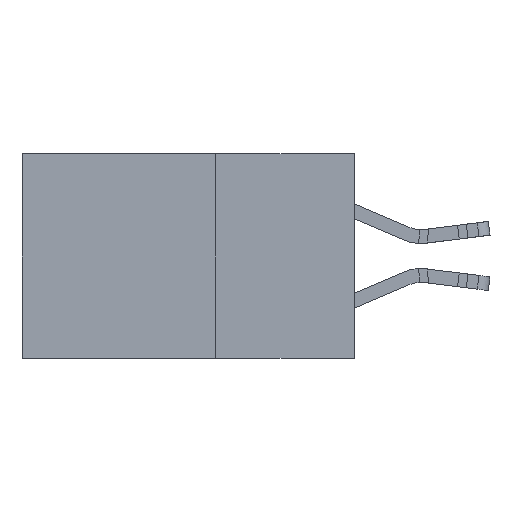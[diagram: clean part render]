
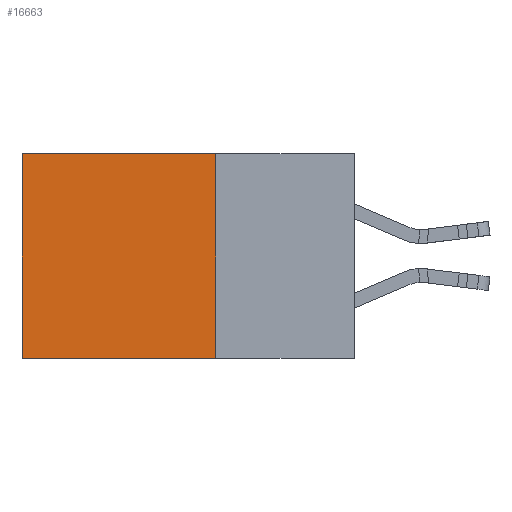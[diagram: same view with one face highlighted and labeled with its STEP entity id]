
A CAD part, left-side view. The second image highlights one B-rep face of the part: STEP entity #16663.
In plain terms, the highlighted planar face has unit normal (-1, 0, 0).
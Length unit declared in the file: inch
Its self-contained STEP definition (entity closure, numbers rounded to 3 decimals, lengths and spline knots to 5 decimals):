
#242 = VERTEX_POINT ( 'NONE', #12766 ) ;
#516 = DIRECTION ( 'NONE',  ( 0., 0., -1. ) ) ;
#1261 = LINE ( 'NONE', #14222, #22498 ) ;
#1479 = DIRECTION ( 'NONE',  ( 0., 0., -1. ) ) ;
#1963 = VECTOR ( 'NONE', #5685, 39.37008 ) ;
#3365 = FACE_OUTER_BOUND ( 'NONE', #12067, .T. ) ;
#3487 = CARTESIAN_POINT ( 'NONE',  ( 0.2615, 0.25, -0.37 ) ) ;
#3983 = EDGE_CURVE ( 'NONE', #13902, #20471, #5508, .T. ) ;
#5508 = LINE ( 'NONE', #19855, #7546 ) ;
#5685 = DIRECTION ( 'NONE',  ( 0., 1., 0. ) ) ;
#6141 = AXIS2_PLACEMENT_3D ( 'NONE', #3487, #16560, #1479 ) ;
#6153 = CARTESIAN_POINT ( 'NONE',  ( 0.2615, 0.6, -0.37 ) ) ;
#7269 = PLANE ( 'NONE',  #6141 ) ;
#7455 = LINE ( 'NONE', #9456, #1963 ) ;
#7546 = VECTOR ( 'NONE', #18314, 39.37008 ) ;
#8210 = LINE ( 'NONE', #17981, #14396 ) ;
#9023 = EDGE_CURVE ( 'NONE', #242, #16367, #7455, .T. ) ;
#9061 = EDGE_CURVE ( 'NONE', #13902, #242, #8210, .T. ) ;
#9456 = CARTESIAN_POINT ( 'NONE',  ( 0.2615, 0.25, -0.37 ) ) ;
#12067 = EDGE_LOOP ( 'NONE', ( #21824, #14579, #18912, #21619 ) ) ;
#12232 = CARTESIAN_POINT ( 'NONE',  ( 0.2615, 0.25, 0. ) ) ;
#12766 = CARTESIAN_POINT ( 'NONE',  ( 0.2615, 0.25, -0.37 ) ) ;
#13902 = VERTEX_POINT ( 'NONE', #12232 ) ;
#14077 = EDGE_CURVE ( 'NONE', #20471, #16367, #1261, .T. ) ;
#14222 = CARTESIAN_POINT ( 'NONE',  ( 0.2615, 0.6, -0.37 ) ) ;
#14396 = VECTOR ( 'NONE', #516, 39.37008 ) ;
#14579 = ORIENTED_EDGE ( 'NONE', *, *, #9023, .F. ) ;
#16367 = VERTEX_POINT ( 'NONE', #6153 ) ;
#16560 = DIRECTION ( 'NONE',  ( 1., 0., 0. ) ) ;
#16663 = ADVANCED_FACE ( 'NONE', ( #3365 ), #7269, .F. ) ;
#17981 = CARTESIAN_POINT ( 'NONE',  ( 0.2615, 0.25, -0.37 ) ) ;
#18314 = DIRECTION ( 'NONE',  ( 0., 1., 0. ) ) ;
#18912 = ORIENTED_EDGE ( 'NONE', *, *, #9061, .F. ) ;
#19855 = CARTESIAN_POINT ( 'NONE',  ( 0.2615, 0.25, 0. ) ) ;
#20471 = VERTEX_POINT ( 'NONE', #22443 ) ;
#21619 = ORIENTED_EDGE ( 'NONE', *, *, #3983, .T. ) ;
#21824 = ORIENTED_EDGE ( 'NONE', *, *, #14077, .T. ) ;
#21866 = DIRECTION ( 'NONE',  ( 0., 0., -1. ) ) ;
#22443 = CARTESIAN_POINT ( 'NONE',  ( 0.2615, 0.6, 0. ) ) ;
#22498 = VECTOR ( 'NONE', #21866, 39.37008 ) ;
